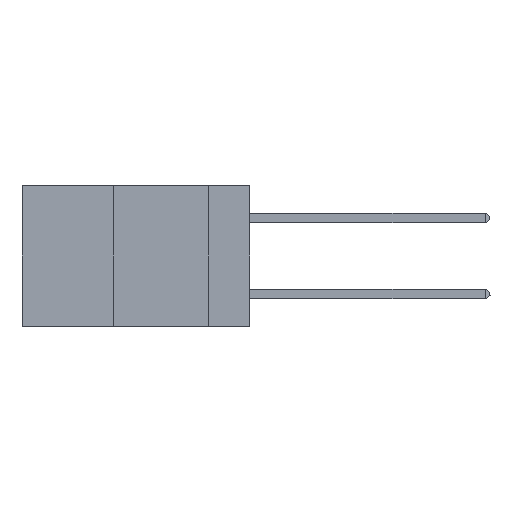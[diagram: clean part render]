
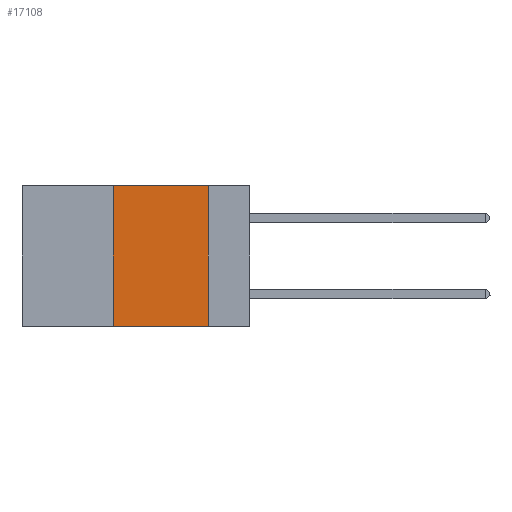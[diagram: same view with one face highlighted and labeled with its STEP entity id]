
A CAD part, left-side view. The second image highlights one B-rep face of the part: STEP entity #17108.
In plain terms, the highlighted planar face has unit normal (-1, 0, 0).
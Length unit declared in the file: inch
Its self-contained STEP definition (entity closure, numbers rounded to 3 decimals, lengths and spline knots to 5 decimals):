
#170 = EDGE_CURVE ( 'NONE', #6319, #9078, #6995, .T. ) ;
#644 = PLANE ( 'NONE',  #24601 ) ;
#906 = ORIENTED_EDGE ( 'NONE', *, *, #23999, .T. ) ;
#915 = DIRECTION ( 'NONE',  ( 0., 0., -1. ) ) ;
#1098 = DIRECTION ( 'NONE',  ( 0., 0., 1. ) ) ;
#2146 = CARTESIAN_POINT ( 'NONE',  ( 0., 0.6, -0.37 ) ) ;
#2579 = DIRECTION ( 'NONE',  ( 1., 0., 0. ) ) ;
#3876 = LINE ( 'NONE', #6387, #25871 ) ;
#4095 = VERTEX_POINT ( 'NONE', #23228 ) ;
#6137 = ORIENTED_EDGE ( 'NONE', *, *, #170, .F. ) ;
#6319 = VERTEX_POINT ( 'NONE', #22576 ) ;
#6387 = CARTESIAN_POINT ( 'NONE',  ( 0., 0.6, 0. ) ) ;
#6995 = LINE ( 'NONE', #15350, #12613 ) ;
#9078 = VERTEX_POINT ( 'NONE', #16783 ) ;
#9253 = ORIENTED_EDGE ( 'NONE', *, *, #11025, .F. ) ;
#11025 = EDGE_CURVE ( 'NONE', #19275, #6319, #3876, .T. ) ;
#11189 = DIRECTION ( 'NONE',  ( 0., 0., -1. ) ) ;
#11831 = FACE_OUTER_BOUND ( 'NONE', #19445, .T. ) ;
#12613 = VECTOR ( 'NONE', #11189, 39.37008 ) ;
#13345 = ORIENTED_EDGE ( 'NONE', *, *, #14392, .F. ) ;
#14392 = EDGE_CURVE ( 'NONE', #4095, #19275, #20692, .T. ) ;
#15257 = VECTOR ( 'NONE', #20870, 39.37008 ) ;
#15259 = CARTESIAN_POINT ( 'NONE',  ( 0., 0.36, 0. ) ) ;
#15350 = CARTESIAN_POINT ( 'NONE',  ( 0., 0.11, 0. ) ) ;
#16783 = CARTESIAN_POINT ( 'NONE',  ( 0., 0.11, -0.37 ) ) ;
#17108 = ADVANCED_FACE ( 'NONE', ( #11831 ), #644, .F. ) ;
#17779 = LINE ( 'NONE', #2146, #15257 ) ;
#19275 = VERTEX_POINT ( 'NONE', #15259 ) ;
#19445 = EDGE_LOOP ( 'NONE', ( #6137, #9253, #13345, #906 ) ) ;
#20692 = LINE ( 'NONE', #25956, #21009 ) ;
#20870 = DIRECTION ( 'NONE',  ( 0., -1., 0. ) ) ;
#21009 = VECTOR ( 'NONE', #1098, 39.37008 ) ;
#22410 = DIRECTION ( 'NONE',  ( 0., -1., 0. ) ) ;
#22576 = CARTESIAN_POINT ( 'NONE',  ( 0., 0.11, 0. ) ) ;
#23228 = CARTESIAN_POINT ( 'NONE',  ( 0., 0.36, -0.37 ) ) ;
#23999 = EDGE_CURVE ( 'NONE', #4095, #9078, #17779, .T. ) ;
#24601 = AXIS2_PLACEMENT_3D ( 'NONE', #24895, #2579, #915 ) ;
#24895 = CARTESIAN_POINT ( 'NONE',  ( 0., 0.6, 0. ) ) ;
#25871 = VECTOR ( 'NONE', #22410, 39.37008 ) ;
#25956 = CARTESIAN_POINT ( 'NONE',  ( 0., 0.36, 0. ) ) ;
